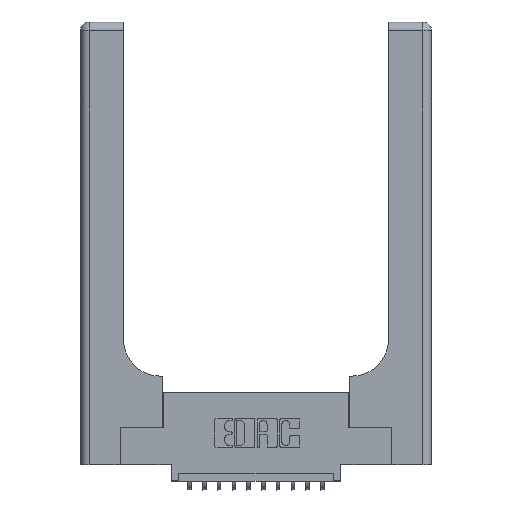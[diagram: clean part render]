
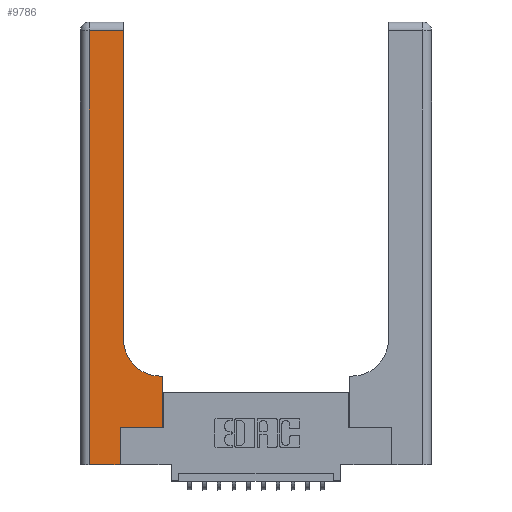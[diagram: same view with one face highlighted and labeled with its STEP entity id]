
A CAD part, top view. The second image highlights one B-rep face of the part: STEP entity #9786.
In plain terms, the highlighted planar face has unit normal (0, 0, 1).
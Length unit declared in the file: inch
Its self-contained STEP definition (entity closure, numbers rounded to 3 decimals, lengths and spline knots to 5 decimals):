
#264 = EDGE_CURVE ( 'NONE', #5456, #4567, #10890, .T. ) ;
#412 = VECTOR ( 'NONE', #1160, 39.37008 ) ;
#494 = LINE ( 'NONE', #14486, #8691 ) ;
#726 = CARTESIAN_POINT ( 'NONE',  ( 0.269, 0.25, 0.37 ) ) ;
#1160 = DIRECTION ( 'NONE',  ( 0., 1., 0. ) ) ;
#1792 = VECTOR ( 'NONE', #10249, 39.37008 ) ;
#1840 = VERTEX_POINT ( 'NONE', #1936 ) ;
#1922 = LINE ( 'NONE', #4535, #15881 ) ;
#1936 = CARTESIAN_POINT ( 'NONE',  ( 0.2915, 0.85, 0.37 ) ) ;
#2207 = FACE_OUTER_BOUND ( 'NONE', #9981, .T. ) ;
#2449 = EDGE_CURVE ( 'NONE', #1840, #12196, #494, .T. ) ;
#2476 = ORIENTED_EDGE ( 'NONE', *, *, #11590, .T. ) ;
#2735 = ORIENTED_EDGE ( 'NONE', *, *, #3879, .T. ) ;
#2795 = DIRECTION ( 'NONE',  ( 1., 0., 0. ) ) ;
#2923 = CARTESIAN_POINT ( 'NONE',  ( 0.5585, 0.25, 0.37 ) ) ;
#3227 = EDGE_CURVE ( 'NONE', #4567, #6814, #11342, .T. ) ;
#3426 = EDGE_CURVE ( 'NONE', #13603, #1840, #14454, .T. ) ;
#3879 = EDGE_CURVE ( 'NONE', #11662, #8079, #4636, .T. ) ;
#4535 = CARTESIAN_POINT ( 'NONE',  ( 0., 2.94, 0.37 ) ) ;
#4546 = EDGE_CURVE ( 'NONE', #8079, #12890, #8831, .T. ) ;
#4567 = VERTEX_POINT ( 'NONE', #11272 ) ;
#4636 = LINE ( 'NONE', #5255, #9260 ) ;
#4975 = LINE ( 'NONE', #6362, #11227 ) ;
#5088 = DIRECTION ( 'NONE',  ( 1., 0., 0. ) ) ;
#5255 = CARTESIAN_POINT ( 'NONE',  ( 0.269, 0.25, 0.37 ) ) ;
#5456 = VERTEX_POINT ( 'NONE', #13886 ) ;
#5496 = VECTOR ( 'NONE', #2795, 39.37008 ) ;
#5703 = DIRECTION ( 'NONE',  ( 0., -1., 0. ) ) ;
#6362 = CARTESIAN_POINT ( 'NONE',  ( 0.2915, 0.6, 0.37 ) ) ;
#6602 = EDGE_CURVE ( 'NONE', #12890, #13603, #4975, .T. ) ;
#6814 = VERTEX_POINT ( 'NONE', #10154 ) ;
#7289 = CARTESIAN_POINT ( 'NONE',  ( 0.2915, 2.94, 0.37 ) ) ;
#7371 = VECTOR ( 'NONE', #5703, 39.37008 ) ;
#8079 = VERTEX_POINT ( 'NONE', #12815 ) ;
#8321 = AXIS2_PLACEMENT_3D ( 'NONE', #11737, #13073, #5088 ) ;
#8521 = LINE ( 'NONE', #12735, #1792 ) ;
#8587 = CARTESIAN_POINT ( 'NONE',  ( 0.06, 3., 0.37 ) ) ;
#8691 = VECTOR ( 'NONE', #13046, 39.37008 ) ;
#8831 = LINE ( 'NONE', #2923, #412 ) ;
#8925 = ORIENTED_EDGE ( 'NONE', *, *, #4546, .T. ) ;
#9260 = VECTOR ( 'NONE', #16193, 39.37008 ) ;
#9393 = CARTESIAN_POINT ( 'NONE',  ( 0.5415, 0.6, 0.37 ) ) ;
#9473 = CARTESIAN_POINT ( 'NONE',  ( 0., 0., 0.37 ) ) ;
#9736 = ORIENTED_EDGE ( 'NONE', *, *, #3426, .T. ) ;
#9786 = ADVANCED_FACE ( 'NONE', ( #2207 ), #14537, .F. ) ;
#9981 = EDGE_LOOP ( 'NONE', ( #15795, #2476, #10517, #10940, #15995, #2735, #8925, #12529, #9736 ) ) ;
#10154 = CARTESIAN_POINT ( 'NONE',  ( 0.269, 0., 0.37 ) ) ;
#10249 = DIRECTION ( 'NONE',  ( 0., 1., 0. ) ) ;
#10479 = CARTESIAN_POINT ( 'NONE',  ( 0., 3., 0.37 ) ) ;
#10517 = ORIENTED_EDGE ( 'NONE', *, *, #264, .T. ) ;
#10890 = LINE ( 'NONE', #8587, #7371 ) ;
#10940 = ORIENTED_EDGE ( 'NONE', *, *, #3227, .T. ) ;
#11227 = VECTOR ( 'NONE', #15653, 39.37008 ) ;
#11272 = CARTESIAN_POINT ( 'NONE',  ( 0.06, 0., 0.37 ) ) ;
#11342 = LINE ( 'NONE', #9473, #5496 ) ;
#11590 = EDGE_CURVE ( 'NONE', #12196, #5456, #1922, .T. ) ;
#11662 = VERTEX_POINT ( 'NONE', #726 ) ;
#11737 = CARTESIAN_POINT ( 'NONE',  ( 0.5415, 0.85, 0.37 ) ) ;
#11738 = CARTESIAN_POINT ( 'NONE',  ( 0.5585, 0.6, 0.37 ) ) ;
#12196 = VERTEX_POINT ( 'NONE', #7289 ) ;
#12529 = ORIENTED_EDGE ( 'NONE', *, *, #6602, .T. ) ;
#12735 = CARTESIAN_POINT ( 'NONE',  ( 0.269, 0., 0.37 ) ) ;
#12815 = CARTESIAN_POINT ( 'NONE',  ( 0.5585, 0.25, 0.37 ) ) ;
#12890 = VERTEX_POINT ( 'NONE', #11738 ) ;
#13046 = DIRECTION ( 'NONE',  ( 0., 1., 0. ) ) ;
#13073 = DIRECTION ( 'NONE',  ( 0., 0., -1. ) ) ;
#13489 = AXIS2_PLACEMENT_3D ( 'NONE', #10479, #17158, #14481 ) ;
#13603 = VERTEX_POINT ( 'NONE', #9393 ) ;
#13886 = CARTESIAN_POINT ( 'NONE',  ( 0.06, 2.94, 0.37 ) ) ;
#14454 = CIRCLE ( 'NONE', #8321, 0.25 ) ;
#14481 = DIRECTION ( 'NONE',  ( -1., 0., 0. ) ) ;
#14486 = CARTESIAN_POINT ( 'NONE',  ( 0.2915, 3., 0.37 ) ) ;
#14537 = PLANE ( 'NONE',  #13489 ) ;
#14789 = EDGE_CURVE ( 'NONE', #6814, #11662, #8521, .T. ) ;
#15653 = DIRECTION ( 'NONE',  ( -1., 0., 0. ) ) ;
#15795 = ORIENTED_EDGE ( 'NONE', *, *, #2449, .T. ) ;
#15881 = VECTOR ( 'NONE', #16635, 39.37008 ) ;
#15995 = ORIENTED_EDGE ( 'NONE', *, *, #14789, .T. ) ;
#16193 = DIRECTION ( 'NONE',  ( 1., 0., 0. ) ) ;
#16635 = DIRECTION ( 'NONE',  ( -1., 0., 0. ) ) ;
#17158 = DIRECTION ( 'NONE',  ( 0., 0., -1. ) ) ;
